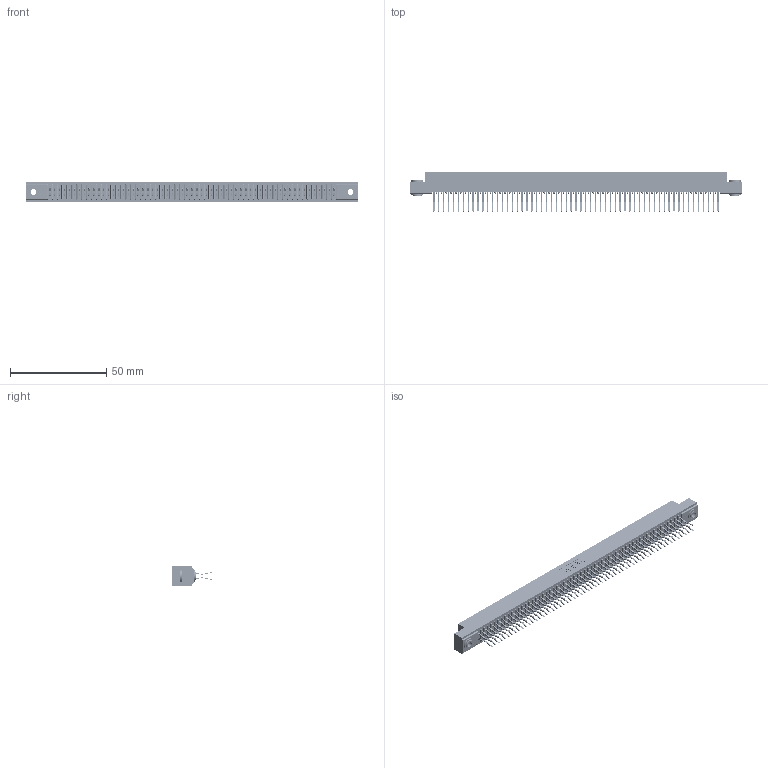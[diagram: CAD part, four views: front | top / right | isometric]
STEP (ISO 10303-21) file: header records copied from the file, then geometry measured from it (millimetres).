
FILE_DESCRIPTION (( 'STEP AP203' ), '1' );
FILE_NAME ('341-118-560-203.STEP', '2018-08-08T14:38:13', ( '' ), ( '' ), 'SwSTEP 2.0', 'SolidWorks 2016', '' );
FILE_SCHEMA (( 'CONFIG_CONTROL_DESIGN' ));
Length unit declared in the file: inch
Products named in the file (4): 341 Part_.156 (3.96) Dia Mounting Holes; 341-292-001_341-292-160; 345-250-002_345-250-002-102; 341-118-560-203
Assembly tree (121 placements, depth 2):
  341-118-560-203
    341 Part_.156 (3.96) Dia Mounting Holes
    341-292-001_341-292-160  x118
    345-250-002_345-250-002-102  x2
Bounding box: 172.09 x 20.37 x 10.16 mm (x, y, z)
Volume: 12841.1 mm3; surface area: 24448.9 mm2
Topology: 121 solids, 121 shells, 8428 faces, 24441 edges, 15854 vertices
Faces by surface type: plane 4812, cylinder 3372, sphere 120, torus 116, cone 8
Entity records: 70343 total; most frequent: CARTESIAN_POINT 11674, ORIENTED_EDGE 11594, DIRECTION 11337, EDGE_CURVE 5797, VECTOR 4687, LINE 4687, VERTEX_POINT 3662, AXIS2_PLACEMENT_3D 3325
